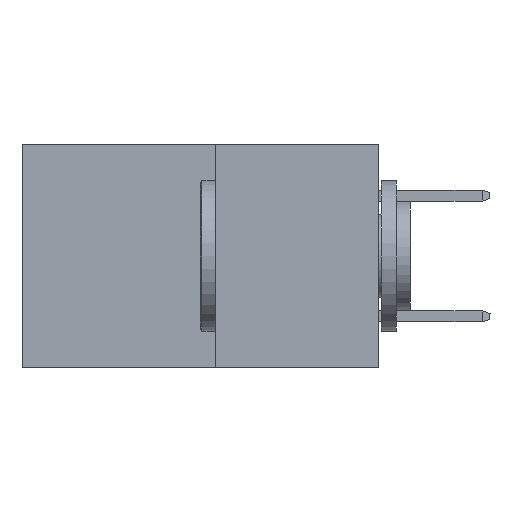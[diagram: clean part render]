
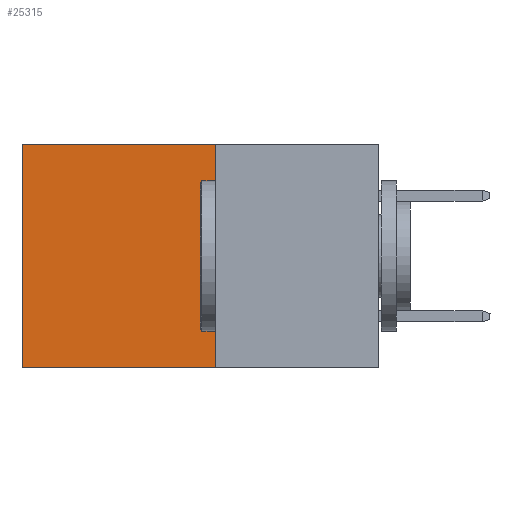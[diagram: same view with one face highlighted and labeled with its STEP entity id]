
A CAD part, left-side view. The second image highlights one B-rep face of the part: STEP entity #25315.
In plain terms, the highlighted planar face has unit normal (-1, 0, 0).
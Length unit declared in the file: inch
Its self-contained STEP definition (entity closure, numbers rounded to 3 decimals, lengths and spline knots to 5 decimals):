
#1527 = VECTOR ( 'NONE', #1819, 39.37008 ) ;
#1819 = DIRECTION ( 'NONE',  ( 0., 0., -1. ) ) ;
#3414 = EDGE_LOOP ( 'NONE', ( #23129, #4793, #19671, #10687 ) ) ;
#3451 = LINE ( 'NONE', #26012, #29943 ) ;
#4793 = ORIENTED_EDGE ( 'NONE', *, *, #22897, .F. ) ;
#7712 = CARTESIAN_POINT ( 'NONE',  ( 0.277, 0.27, -0.37 ) ) ;
#8506 = DIRECTION ( 'NONE',  ( 0., 1., 0. ) ) ;
#8520 = DIRECTION ( 'NONE',  ( 0., 0., -1. ) ) ;
#8883 = LINE ( 'NONE', #15531, #1527 ) ;
#9076 = EDGE_CURVE ( 'NONE', #21400, #32917, #13186, .T. ) ;
#10687 = ORIENTED_EDGE ( 'NONE', *, *, #30771, .T. ) ;
#11092 = LINE ( 'NONE', #24848, #31934 ) ;
#12274 = VERTEX_POINT ( 'NONE', #18177 ) ;
#13186 = LINE ( 'NONE', #27594, #34816 ) ;
#14158 = CARTESIAN_POINT ( 'NONE',  ( 0.277, 0.59, -0.37 ) ) ;
#15531 = CARTESIAN_POINT ( 'NONE',  ( 0.277, 0.27, -0.37 ) ) ;
#15893 = CARTESIAN_POINT ( 'NONE',  ( 0.277, 0.27, -0.37 ) ) ;
#18177 = CARTESIAN_POINT ( 'NONE',  ( 0.277, 0.27, 0. ) ) ;
#18610 = DIRECTION ( 'NONE',  ( 0., 0., -1. ) ) ;
#19671 = ORIENTED_EDGE ( 'NONE', *, *, #25221, .F. ) ;
#21400 = VERTEX_POINT ( 'NONE', #25636 ) ;
#22897 = EDGE_CURVE ( 'NONE', #27882, #32917, #3451, .T. ) ;
#23129 = ORIENTED_EDGE ( 'NONE', *, *, #9076, .T. ) ;
#24848 = CARTESIAN_POINT ( 'NONE',  ( 0.277, 0.27, 0. ) ) ;
#25221 = EDGE_CURVE ( 'NONE', #12274, #27882, #8883, .T. ) ;
#25315 = ADVANCED_FACE ( 'NONE', ( #28065 ), #29435, .F. ) ;
#25636 = CARTESIAN_POINT ( 'NONE',  ( 0.277, 0.59, 0. ) ) ;
#26012 = CARTESIAN_POINT ( 'NONE',  ( 0.277, 0.27, -0.37 ) ) ;
#26373 = AXIS2_PLACEMENT_3D ( 'NONE', #15893, #34836, #18610 ) ;
#27594 = CARTESIAN_POINT ( 'NONE',  ( 0.277, 0.59, -0.37 ) ) ;
#27882 = VERTEX_POINT ( 'NONE', #7712 ) ;
#28065 = FACE_OUTER_BOUND ( 'NONE', #3414, .T. ) ;
#28742 = DIRECTION ( 'NONE',  ( 0., 1., 0. ) ) ;
#29435 = PLANE ( 'NONE',  #26373 ) ;
#29943 = VECTOR ( 'NONE', #28742, 39.37008 ) ;
#30771 = EDGE_CURVE ( 'NONE', #12274, #21400, #11092, .T. ) ;
#31934 = VECTOR ( 'NONE', #8506, 39.37008 ) ;
#32917 = VERTEX_POINT ( 'NONE', #14158 ) ;
#34816 = VECTOR ( 'NONE', #8520, 39.37008 ) ;
#34836 = DIRECTION ( 'NONE',  ( 1., 0., 0. ) ) ;
